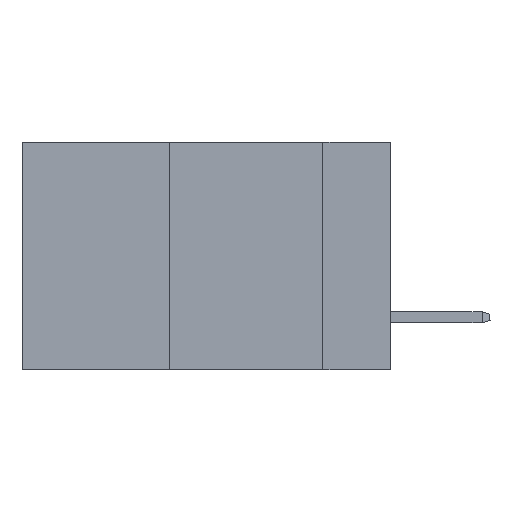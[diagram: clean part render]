
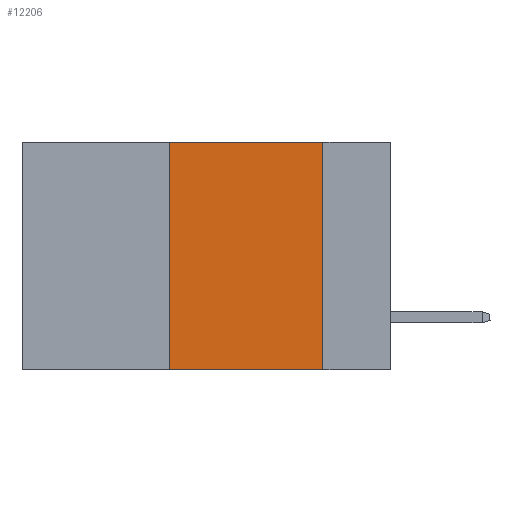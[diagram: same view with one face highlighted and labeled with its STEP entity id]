
A CAD part, left-side view. The second image highlights one B-rep face of the part: STEP entity #12206.
In plain terms, the highlighted planar face has unit normal (-1, 0, 0).
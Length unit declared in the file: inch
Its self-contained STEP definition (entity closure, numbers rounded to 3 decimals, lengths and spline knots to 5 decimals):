
#9 = EDGE_CURVE ( 'NONE', #1143, #10063, #7059, .T. ) ;
#113 = CARTESIAN_POINT ( 'NONE',  ( 0., 0.36, 0. ) ) ;
#173 = CARTESIAN_POINT ( 'NONE',  ( 0., 0.11, 0. ) ) ;
#558 = VECTOR ( 'NONE', #5867, 39.37008 ) ;
#740 = CARTESIAN_POINT ( 'NONE',  ( 0., 0.11, -0.37 ) ) ;
#1143 = VERTEX_POINT ( 'NONE', #8557 ) ;
#1482 = DIRECTION ( 'NONE',  ( 0., 0., -1. ) ) ;
#2806 = LINE ( 'NONE', #113, #558 ) ;
#2822 = CARTESIAN_POINT ( 'NONE',  ( 0., 0.6, -0.37 ) ) ;
#2938 = EDGE_CURVE ( 'NONE', #10324, #10063, #6750, .T. ) ;
#3799 = CARTESIAN_POINT ( 'NONE',  ( 0., 0.11, 0. ) ) ;
#3815 = EDGE_CURVE ( 'NONE', #7489, #10324, #11161, .T. ) ;
#4140 = AXIS2_PLACEMENT_3D ( 'NONE', #4214, #11078, #9008 ) ;
#4214 = CARTESIAN_POINT ( 'NONE',  ( 0., 0.6, 0. ) ) ;
#4992 = CARTESIAN_POINT ( 'NONE',  ( 0., 0.6, 0. ) ) ;
#5365 = CARTESIAN_POINT ( 'NONE',  ( 0., 0.36, 0. ) ) ;
#5867 = DIRECTION ( 'NONE',  ( 0., 0., 1. ) ) ;
#5980 = VECTOR ( 'NONE', #1482, 39.37008 ) ;
#6567 = ORIENTED_EDGE ( 'NONE', *, *, #10690, .F. ) ;
#6750 = LINE ( 'NONE', #173, #5980 ) ;
#6809 = ORIENTED_EDGE ( 'NONE', *, *, #2938, .F. ) ;
#7059 = LINE ( 'NONE', #2822, #9811 ) ;
#7094 = EDGE_LOOP ( 'NONE', ( #6809, #9125, #6567, #8845 ) ) ;
#7489 = VERTEX_POINT ( 'NONE', #5365 ) ;
#7823 = FACE_OUTER_BOUND ( 'NONE', #7094, .T. ) ;
#8044 = PLANE ( 'NONE',  #4140 ) ;
#8541 = VECTOR ( 'NONE', #9976, 39.37008 ) ;
#8557 = CARTESIAN_POINT ( 'NONE',  ( 0., 0.36, -0.37 ) ) ;
#8845 = ORIENTED_EDGE ( 'NONE', *, *, #9, .T. ) ;
#9008 = DIRECTION ( 'NONE',  ( 0., 0., -1. ) ) ;
#9125 = ORIENTED_EDGE ( 'NONE', *, *, #3815, .F. ) ;
#9811 = VECTOR ( 'NONE', #11627, 39.37008 ) ;
#9976 = DIRECTION ( 'NONE',  ( 0., -1., 0. ) ) ;
#10063 = VERTEX_POINT ( 'NONE', #740 ) ;
#10324 = VERTEX_POINT ( 'NONE', #3799 ) ;
#10690 = EDGE_CURVE ( 'NONE', #1143, #7489, #2806, .T. ) ;
#11078 = DIRECTION ( 'NONE',  ( 1., 0., 0. ) ) ;
#11161 = LINE ( 'NONE', #4992, #8541 ) ;
#11627 = DIRECTION ( 'NONE',  ( 0., -1., 0. ) ) ;
#12206 = ADVANCED_FACE ( 'NONE', ( #7823 ), #8044, .F. ) ;
